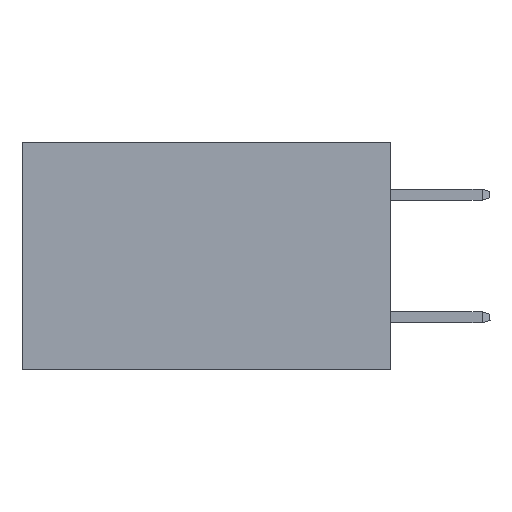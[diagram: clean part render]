
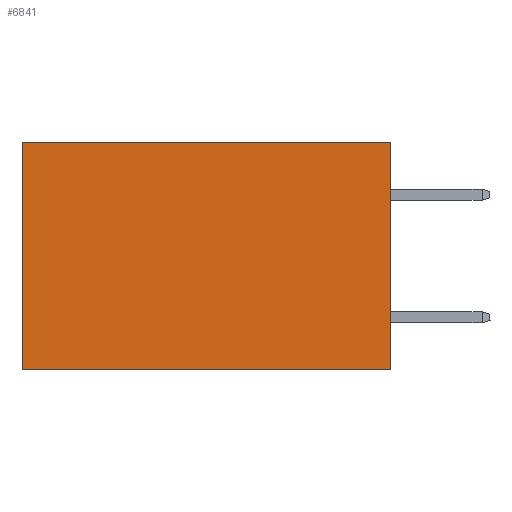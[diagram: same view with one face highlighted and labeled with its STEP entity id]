
A CAD part, left-side view. The second image highlights one B-rep face of the part: STEP entity #6841.
In plain terms, the highlighted planar face has unit normal (-1, 0, 0).
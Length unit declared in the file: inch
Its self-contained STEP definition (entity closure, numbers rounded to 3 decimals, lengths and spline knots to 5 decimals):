
#127 = CARTESIAN_POINT ( 'NONE',  ( 0.2875, 0., 0. ) ) ;
#260 = CARTESIAN_POINT ( 'NONE',  ( 0.2875, 0., 0. ) ) ;
#580 = ORIENTED_EDGE ( 'NONE', *, *, #4246, .F. ) ;
#687 = DIRECTION ( 'NONE',  ( 0., 1., 0. ) ) ;
#790 = ORIENTED_EDGE ( 'NONE', *, *, #2831, .T. ) ;
#1297 = LINE ( 'NONE', #9934, #10894 ) ;
#2163 = DIRECTION ( 'NONE',  ( 0., 0., -1. ) ) ;
#2193 = VERTEX_POINT ( 'NONE', #9955 ) ;
#2769 = EDGE_LOOP ( 'NONE', ( #790, #8285, #580, #8686 ) ) ;
#2831 = EDGE_CURVE ( 'NONE', #10134, #3449, #11947, .T. ) ;
#2999 = LINE ( 'NONE', #4542, #7598 ) ;
#3449 = VERTEX_POINT ( 'NONE', #7746 ) ;
#3481 = AXIS2_PLACEMENT_3D ( 'NONE', #260, #4111, #5629 ) ;
#4111 = DIRECTION ( 'NONE',  ( 1., 0., 0. ) ) ;
#4183 = VECTOR ( 'NONE', #687, 39.37008 ) ;
#4246 = EDGE_CURVE ( 'NONE', #2193, #11685, #1297, .T. ) ;
#4514 = DIRECTION ( 'NONE',  ( 0., 1., 0. ) ) ;
#4542 = CARTESIAN_POINT ( 'NONE',  ( 0.2875, 0., -0.37 ) ) ;
#4820 = PLANE ( 'NONE',  #3481 ) ;
#5064 = CARTESIAN_POINT ( 'NONE',  ( 0.2875, 0., -0.37 ) ) ;
#5180 = VECTOR ( 'NONE', #10682, 39.37008 ) ;
#5587 = EDGE_CURVE ( 'NONE', #11685, #3449, #2999, .T. ) ;
#5629 = DIRECTION ( 'NONE',  ( 0., 0., -1. ) ) ;
#5881 = EDGE_CURVE ( 'NONE', #2193, #10134, #7133, .T. ) ;
#6841 = ADVANCED_FACE ( 'NONE', ( #8277 ), #4820, .F. ) ;
#7133 = LINE ( 'NONE', #127, #4183 ) ;
#7598 = VECTOR ( 'NONE', #4514, 39.37008 ) ;
#7746 = CARTESIAN_POINT ( 'NONE',  ( 0.2875, 0.6, -0.37 ) ) ;
#8277 = FACE_OUTER_BOUND ( 'NONE', #2769, .T. ) ;
#8285 = ORIENTED_EDGE ( 'NONE', *, *, #5587, .F. ) ;
#8686 = ORIENTED_EDGE ( 'NONE', *, *, #5881, .T. ) ;
#9934 = CARTESIAN_POINT ( 'NONE',  ( 0.2875, 0., 0. ) ) ;
#9955 = CARTESIAN_POINT ( 'NONE',  ( 0.2875, 0., 0. ) ) ;
#10134 = VERTEX_POINT ( 'NONE', #10552 ) ;
#10552 = CARTESIAN_POINT ( 'NONE',  ( 0.2875, 0.6, 0. ) ) ;
#10600 = CARTESIAN_POINT ( 'NONE',  ( 0.2875, 0.6, 0. ) ) ;
#10682 = DIRECTION ( 'NONE',  ( 0., 0., -1. ) ) ;
#10894 = VECTOR ( 'NONE', #2163, 39.37008 ) ;
#11685 = VERTEX_POINT ( 'NONE', #5064 ) ;
#11947 = LINE ( 'NONE', #10600, #5180 ) ;
